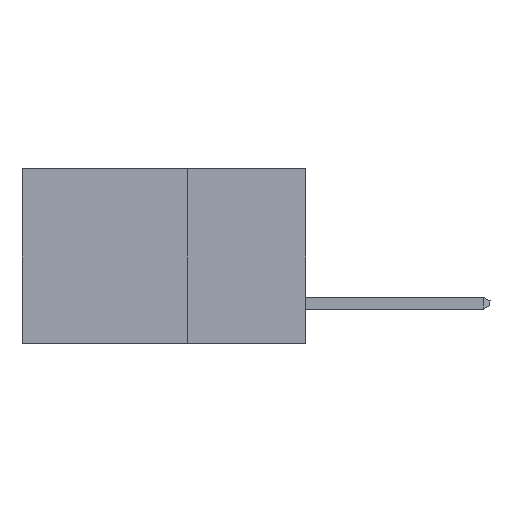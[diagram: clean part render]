
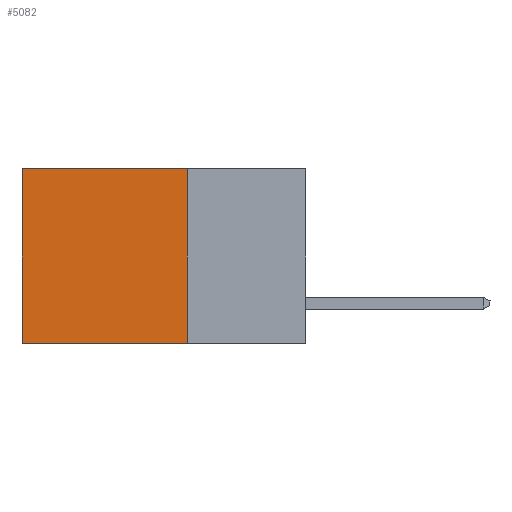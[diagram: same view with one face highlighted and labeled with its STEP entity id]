
A CAD part, left-side view. The second image highlights one B-rep face of the part: STEP entity #5082.
In plain terms, the highlighted planar face has unit normal (-1, 0, 0).
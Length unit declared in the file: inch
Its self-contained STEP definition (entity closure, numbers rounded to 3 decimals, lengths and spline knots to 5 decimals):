
#15 = CARTESIAN_POINT ( 'NONE',  ( 0.2615, 0.25, 0. ) ) ;
#74 = EDGE_CURVE ( 'NONE', #3254, #5023, #6346, .T. ) ;
#331 = CARTESIAN_POINT ( 'NONE',  ( 0.2615, 0.25, -0.37 ) ) ;
#375 = FACE_OUTER_BOUND ( 'NONE', #579, .T. ) ;
#426 = CARTESIAN_POINT ( 'NONE',  ( 0.2615, 0.6, 0. ) ) ;
#435 = DIRECTION ( 'NONE',  ( 0., 0., -1. ) ) ;
#579 = EDGE_LOOP ( 'NONE', ( #4646, #1389, #10225, #3633 ) ) ;
#1127 = VERTEX_POINT ( 'NONE', #6913 ) ;
#1382 = CARTESIAN_POINT ( 'NONE',  ( 0.2615, 0.25, -0.37 ) ) ;
#1389 = ORIENTED_EDGE ( 'NONE', *, *, #7825, .F. ) ;
#1954 = DIRECTION ( 'NONE',  ( 0., 0., -1. ) ) ;
#3106 = EDGE_CURVE ( 'NONE', #3254, #1127, #8264, .T. ) ;
#3254 = VERTEX_POINT ( 'NONE', #7042 ) ;
#3380 = PLANE ( 'NONE',  #5796 ) ;
#3633 = ORIENTED_EDGE ( 'NONE', *, *, #74, .T. ) ;
#3880 = VECTOR ( 'NONE', #4106, 39.37008 ) ;
#3930 = DIRECTION ( 'NONE',  ( 0., 1., 0. ) ) ;
#4106 = DIRECTION ( 'NONE',  ( 0., 1., 0. ) ) ;
#4376 = CARTESIAN_POINT ( 'NONE',  ( 0.2615, 0.6, -0.37 ) ) ;
#4646 = ORIENTED_EDGE ( 'NONE', *, *, #7082, .T. ) ;
#4926 = VERTEX_POINT ( 'NONE', #5573 ) ;
#5023 = VERTEX_POINT ( 'NONE', #426 ) ;
#5082 = ADVANCED_FACE ( 'NONE', ( #375 ), #3380, .F. ) ;
#5138 = VECTOR ( 'NONE', #3930, 39.37008 ) ;
#5573 = CARTESIAN_POINT ( 'NONE',  ( 0.2615, 0.6, -0.37 ) ) ;
#5796 = AXIS2_PLACEMENT_3D ( 'NONE', #331, #6563, #5799 ) ;
#5799 = DIRECTION ( 'NONE',  ( 0., 0., -1. ) ) ;
#5802 = VECTOR ( 'NONE', #435, 39.37008 ) ;
#6226 = LINE ( 'NONE', #1382, #5138 ) ;
#6346 = LINE ( 'NONE', #15, #3880 ) ;
#6563 = DIRECTION ( 'NONE',  ( 1., 0., 0. ) ) ;
#6748 = VECTOR ( 'NONE', #1954, 39.37008 ) ;
#6913 = CARTESIAN_POINT ( 'NONE',  ( 0.2615, 0.25, -0.37 ) ) ;
#6927 = LINE ( 'NONE', #4376, #5802 ) ;
#7042 = CARTESIAN_POINT ( 'NONE',  ( 0.2615, 0.25, 0. ) ) ;
#7082 = EDGE_CURVE ( 'NONE', #5023, #4926, #6927, .T. ) ;
#7825 = EDGE_CURVE ( 'NONE', #1127, #4926, #6226, .T. ) ;
#8264 = LINE ( 'NONE', #9145, #6748 ) ;
#9145 = CARTESIAN_POINT ( 'NONE',  ( 0.2615, 0.25, -0.37 ) ) ;
#10225 = ORIENTED_EDGE ( 'NONE', *, *, #3106, .F. ) ;
